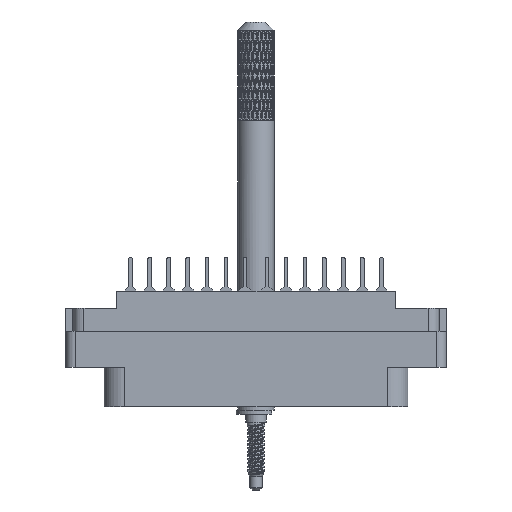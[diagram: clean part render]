
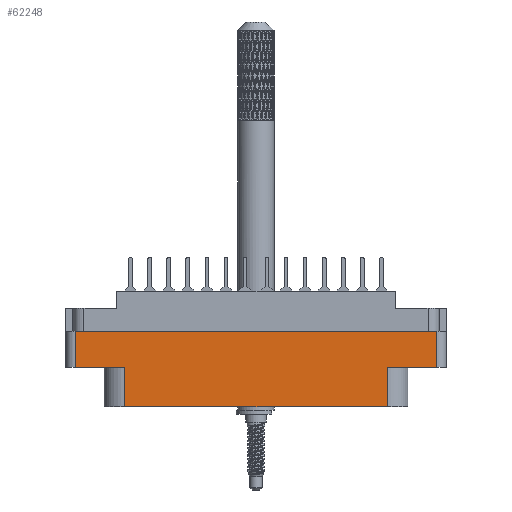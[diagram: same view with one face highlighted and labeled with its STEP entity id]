
A CAD part, front view. The second image highlights one B-rep face of the part: STEP entity #62248.
In plain terms, the highlighted planar face has unit normal (0, -1, 0).
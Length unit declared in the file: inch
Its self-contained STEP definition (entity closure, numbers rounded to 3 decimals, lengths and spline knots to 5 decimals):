
#2780 = VERTEX_POINT ( 'NONE', #35018 ) ;
#3414 = DIRECTION ( 'NONE',  ( -1., 0., 0. ) ) ;
#5242 = EDGE_CURVE ( 'NONE', #18152, #2780, #62847, .T. ) ;
#10014 = VERTEX_POINT ( 'NONE', #27256 ) ;
#10048 = DIRECTION ( 'NONE',  ( 1., 0., 0. ) ) ;
#10859 = VERTEX_POINT ( 'NONE', #92542 ) ;
#11436 = VECTOR ( 'NONE', #10048, 39.37008 ) ;
#14536 = CARTESIAN_POINT ( 'NONE',  ( 0., -0.438, -0.52 ) ) ;
#17765 = EDGE_CURVE ( 'NONE', #36602, #96748, #43337, .T. ) ;
#18152 = VERTEX_POINT ( 'NONE', #82442 ) ;
#18568 = CARTESIAN_POINT ( 'NONE',  ( -1.2955, -0.438, -0.789 ) ) ;
#18603 = EDGE_CURVE ( 'NONE', #10014, #18152, #96139, .T. ) ;
#21665 = VECTOR ( 'NONE', #83957, 39.37008 ) ;
#22733 = VECTOR ( 'NONE', #102738, 39.37008 ) ;
#23957 = ORIENTED_EDGE ( 'NONE', *, *, #26235, .F. ) ;
#23987 = PLANE ( 'NONE',  #32650 ) ;
#26235 = EDGE_CURVE ( 'NONE', #10014, #10859, #92362, .T. ) ;
#27256 = CARTESIAN_POINT ( 'NONE',  ( -0.895, -0.438, -0.52 ) ) ;
#29275 = ORIENTED_EDGE ( 'NONE', *, *, #17765, .T. ) ;
#32184 = ORIENTED_EDGE ( 'NONE', *, *, #5242, .T. ) ;
#32410 = DIRECTION ( 'NONE',  ( 1., 0., 0. ) ) ;
#32650 = AXIS2_PLACEMENT_3D ( 'NONE', #42213, #86657, #104083 ) ;
#33669 = LINE ( 'NONE', #14536, #96255 ) ;
#34628 = CARTESIAN_POINT ( 'NONE',  ( -1.2335, -0.438, -0.274 ) ) ;
#35018 = CARTESIAN_POINT ( 'NONE',  ( 0.895, -0.438, -0.789 ) ) ;
#35937 = VECTOR ( 'NONE', #32410, 39.37008 ) ;
#36411 = CARTESIAN_POINT ( 'NONE',  ( 1.2335, -0.438, -0.789 ) ) ;
#36425 = VECTOR ( 'NONE', #90151, 39.37008 ) ;
#36602 = VERTEX_POINT ( 'NONE', #66957 ) ;
#38394 = VERTEX_POINT ( 'NONE', #34628 ) ;
#41625 = CARTESIAN_POINT ( 'NONE',  ( 0.895, -0.438, -0.52 ) ) ;
#42213 = CARTESIAN_POINT ( 'NONE',  ( -1.2955, -0.438, -0.789 ) ) ;
#43337 = LINE ( 'NONE', #36411, #36425 ) ;
#45662 = EDGE_LOOP ( 'NONE', ( #46675, #72442, #23957, #72737, #32184, #47810, #54227, #29275 ) ) ;
#45875 = EDGE_CURVE ( 'NONE', #38394, #10859, #63345, .T. ) ;
#46675 = ORIENTED_EDGE ( 'NONE', *, *, #94848, .F. ) ;
#47810 = ORIENTED_EDGE ( 'NONE', *, *, #68818, .T. ) ;
#54227 = ORIENTED_EDGE ( 'NONE', *, *, #107768, .F. ) ;
#58025 = CARTESIAN_POINT ( 'NONE',  ( 0., -0.438, -0.274 ) ) ;
#62248 = ADVANCED_FACE ( 'NONE', ( #89134 ), #23987, .T. ) ;
#62847 = LINE ( 'NONE', #18568, #11436 ) ;
#63345 = LINE ( 'NONE', #95923, #21665 ) ;
#66279 = CARTESIAN_POINT ( 'NONE',  ( 0.895, -0.438, -0.52 ) ) ;
#66957 = CARTESIAN_POINT ( 'NONE',  ( 1.2335, -0.438, -0.52 ) ) ;
#68818 = EDGE_CURVE ( 'NONE', #2780, #95788, #95157, .T. ) ;
#72442 = ORIENTED_EDGE ( 'NONE', *, *, #45875, .T. ) ;
#72737 = ORIENTED_EDGE ( 'NONE', *, *, #18603, .T. ) ;
#76649 = VECTOR ( 'NONE', #89750, 39.37008 ) ;
#81914 = CARTESIAN_POINT ( 'NONE',  ( -0.895, -0.438, -0.789 ) ) ;
#82442 = CARTESIAN_POINT ( 'NONE',  ( -0.895, -0.438, -0.789 ) ) ;
#83146 = CARTESIAN_POINT ( 'NONE',  ( 0., -0.438, -0.52 ) ) ;
#83330 = LINE ( 'NONE', #58025, #35937 ) ;
#83957 = DIRECTION ( 'NONE',  ( 0., 0., -1. ) ) ;
#86657 = DIRECTION ( 'NONE',  ( 0., -1., 0. ) ) ;
#89134 = FACE_OUTER_BOUND ( 'NONE', #45662, .T. ) ;
#89750 = DIRECTION ( 'NONE',  ( 0., 0., -1. ) ) ;
#90151 = DIRECTION ( 'NONE',  ( 0., 0., 1. ) ) ;
#92362 = LINE ( 'NONE', #83146, #95095 ) ;
#92542 = CARTESIAN_POINT ( 'NONE',  ( -1.2335, -0.438, -0.52 ) ) ;
#94848 = EDGE_CURVE ( 'NONE', #38394, #96748, #83330, .T. ) ;
#95095 = VECTOR ( 'NONE', #3414, 39.37008 ) ;
#95157 = LINE ( 'NONE', #41625, #22733 ) ;
#95788 = VERTEX_POINT ( 'NONE', #66279 ) ;
#95923 = CARTESIAN_POINT ( 'NONE',  ( -1.2335, -0.438, -0.789 ) ) ;
#96139 = LINE ( 'NONE', #81914, #76649 ) ;
#96255 = VECTOR ( 'NONE', #111823, 39.37008 ) ;
#96748 = VERTEX_POINT ( 'NONE', #99803 ) ;
#99803 = CARTESIAN_POINT ( 'NONE',  ( 1.2335, -0.438, -0.274 ) ) ;
#102738 = DIRECTION ( 'NONE',  ( 0., 0., 1. ) ) ;
#104083 = DIRECTION ( 'NONE',  ( 0., 0., -1. ) ) ;
#107768 = EDGE_CURVE ( 'NONE', #36602, #95788, #33669, .T. ) ;
#111823 = DIRECTION ( 'NONE',  ( -1., 0., 0. ) ) ;
